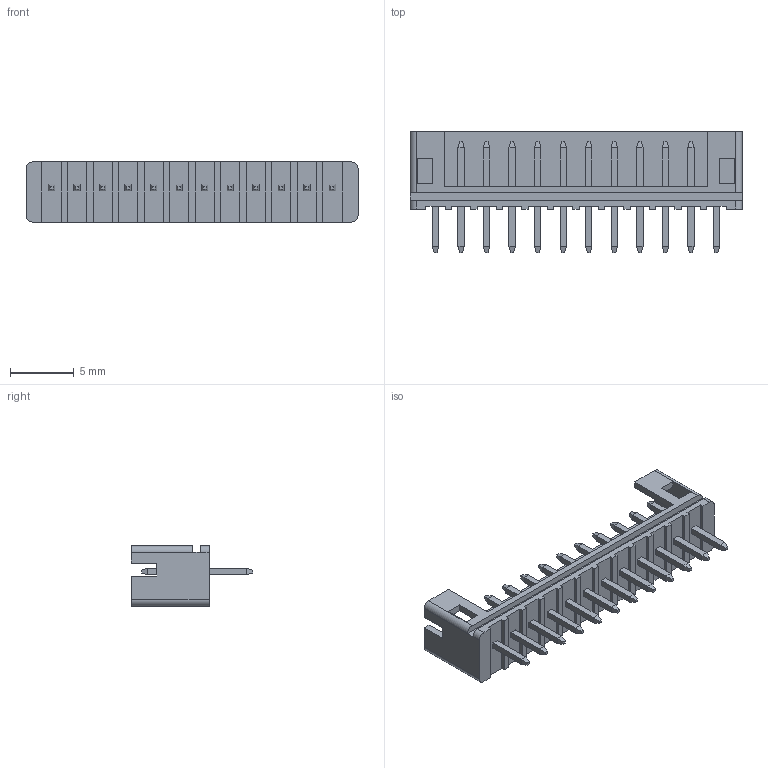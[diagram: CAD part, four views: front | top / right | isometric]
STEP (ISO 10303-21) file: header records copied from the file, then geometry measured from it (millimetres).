
FILE_DESCRIPTION (( 'STEP AP203' ), '1' );
FILE_NAME ('140-512-415-101.STEP', '2020-09-25T11:18:16', ( '' ), ( '' ), 'SwSTEP 2.0', 'SolidWorks 2020', '' );
FILE_SCHEMA (( 'CONFIG_CONTROL_DESIGN' ));
Length unit declared in the file: millimetre
Products named in the file (3): 140-512-415-101; V LI Housing_512; V LI Contact_Str
Assembly tree (13 placements, depth 2):
  140-512-415-101
    V LI Housing_512
    V LI Contact_Str  x12
Bounding box: 26 x 9.5 x 4.7 mm (x, y, z)
Volume: 270.1 mm3; surface area: 986.5 mm2
Topology: 13 solids, 13 shells, 304 faces, 740 edges, 460 vertices
Faces by surface type: plane 298, cylinder 6
Entity records: 5525 total; most frequent: CARTESIAN_POINT 882, ORIENTED_EDGE 864, DIRECTION 776, EDGE_CURVE 432, LINE 420, VECTOR 420, VERTEX_POINT 284, AXIS2_PLACEMENT_3D 178
